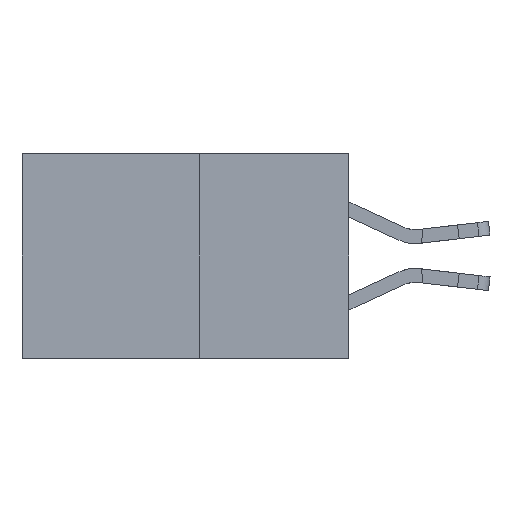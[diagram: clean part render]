
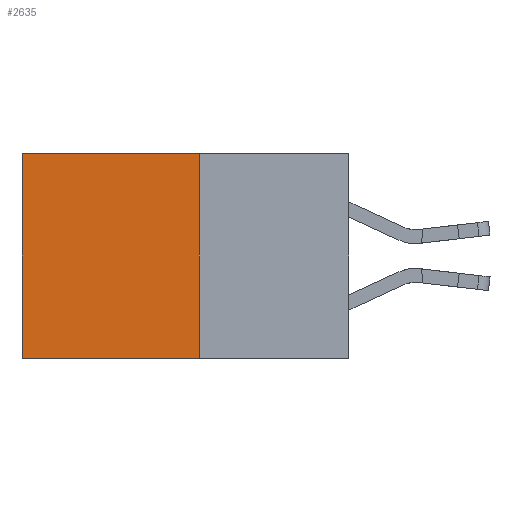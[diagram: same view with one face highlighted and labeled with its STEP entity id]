
A CAD part, left-side view. The second image highlights one B-rep face of the part: STEP entity #2635.
In plain terms, the highlighted planar face has unit normal (-1, 0, 0).
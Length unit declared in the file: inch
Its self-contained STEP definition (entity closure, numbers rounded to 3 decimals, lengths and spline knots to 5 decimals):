
#136 = VECTOR ( 'NONE', #10689, 39.37008 ) ;
#646 = DIRECTION ( 'NONE',  ( 0., 0., -1. ) ) ;
#1177 = CARTESIAN_POINT ( 'NONE',  ( 0.277, 0.27, -0.37 ) ) ;
#2635 = ADVANCED_FACE ( 'NONE', ( #10531 ), #15379, .F. ) ;
#3090 = ORIENTED_EDGE ( 'NONE', *, *, #5103, .T. ) ;
#3148 = CARTESIAN_POINT ( 'NONE',  ( 0.277, 0.27, -0.37 ) ) ;
#3887 = CARTESIAN_POINT ( 'NONE',  ( 0.277, 0.27, 0. ) ) ;
#3994 = VERTEX_POINT ( 'NONE', #7120 ) ;
#5103 = EDGE_CURVE ( 'NONE', #3994, #6483, #10851, .T. ) ;
#5221 = LINE ( 'NONE', #5540, #8709 ) ;
#5540 = CARTESIAN_POINT ( 'NONE',  ( 0.277, 0.27, 0. ) ) ;
#5562 = DIRECTION ( 'NONE',  ( 0., 1., 0. ) ) ;
#5641 = VERTEX_POINT ( 'NONE', #14425 ) ;
#6359 = AXIS2_PLACEMENT_3D ( 'NONE', #3148, #9357, #646 ) ;
#6483 = VERTEX_POINT ( 'NONE', #12641 ) ;
#6615 = ORIENTED_EDGE ( 'NONE', *, *, #15203, .F. ) ;
#6974 = CARTESIAN_POINT ( 'NONE',  ( 0.277, 0.59, -0.37 ) ) ;
#7120 = CARTESIAN_POINT ( 'NONE',  ( 0.277, 0.59, 0. ) ) ;
#7764 = EDGE_CURVE ( 'NONE', #11599, #3994, #5221, .T. ) ;
#8196 = VECTOR ( 'NONE', #5562, 39.37008 ) ;
#8709 = VECTOR ( 'NONE', #12628, 39.37008 ) ;
#8836 = ORIENTED_EDGE ( 'NONE', *, *, #7764, .T. ) ;
#9232 = LINE ( 'NONE', #1177, #136 ) ;
#9357 = DIRECTION ( 'NONE',  ( 1., 0., 0. ) ) ;
#10531 = FACE_OUTER_BOUND ( 'NONE', #14658, .T. ) ;
#10554 = DIRECTION ( 'NONE',  ( 0., 0., -1. ) ) ;
#10689 = DIRECTION ( 'NONE',  ( 0., 0., -1. ) ) ;
#10851 = LINE ( 'NONE', #6974, #11211 ) ;
#11211 = VECTOR ( 'NONE', #10554, 39.37008 ) ;
#11599 = VERTEX_POINT ( 'NONE', #3887 ) ;
#12528 = EDGE_CURVE ( 'NONE', #5641, #6483, #14556, .T. ) ;
#12628 = DIRECTION ( 'NONE',  ( 0., 1., 0. ) ) ;
#12641 = CARTESIAN_POINT ( 'NONE',  ( 0.277, 0.59, -0.37 ) ) ;
#13855 = CARTESIAN_POINT ( 'NONE',  ( 0.277, 0.27, -0.37 ) ) ;
#14425 = CARTESIAN_POINT ( 'NONE',  ( 0.277, 0.27, -0.37 ) ) ;
#14556 = LINE ( 'NONE', #13855, #8196 ) ;
#14658 = EDGE_LOOP ( 'NONE', ( #3090, #15082, #6615, #8836 ) ) ;
#15082 = ORIENTED_EDGE ( 'NONE', *, *, #12528, .F. ) ;
#15203 = EDGE_CURVE ( 'NONE', #11599, #5641, #9232, .T. ) ;
#15379 = PLANE ( 'NONE',  #6359 ) ;
